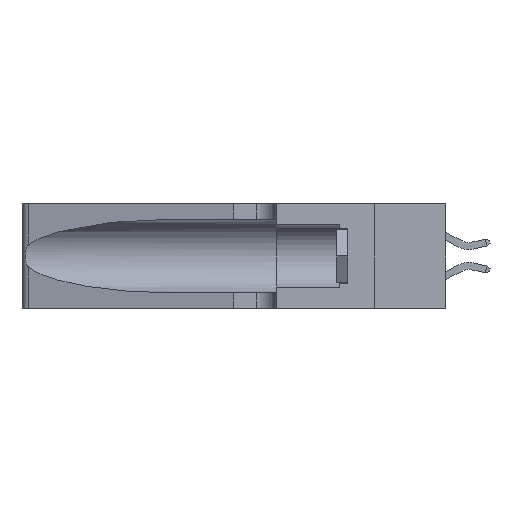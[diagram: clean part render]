
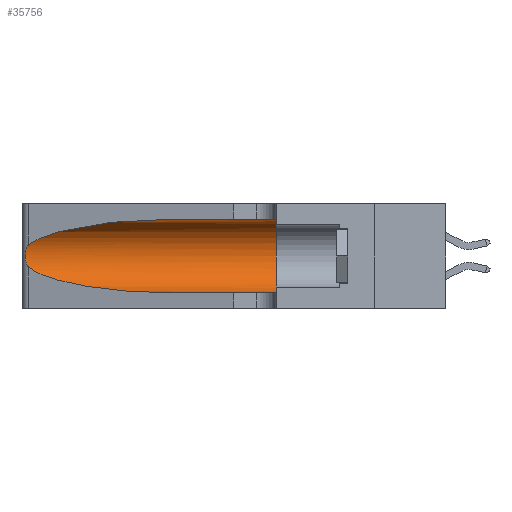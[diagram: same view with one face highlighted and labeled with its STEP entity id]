
A CAD part, left-side view. The second image highlights one B-rep face of the part: STEP entity #35756.
In plain terms, the highlighted cylindrical face has radius 3.308 mm (diameter 6.617 mm), a partial arc.
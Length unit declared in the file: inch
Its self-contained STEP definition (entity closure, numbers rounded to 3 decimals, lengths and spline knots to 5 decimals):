
#1296 = CARTESIAN_POINT ( 'NONE',  ( 0.1305, 0.35, 0.05475 ) ) ;
#1552 = AXIS2_PLACEMENT_3D ( 'NONE', #14078, #30241, #23945 ) ;
#2430 = CIRCLE ( 'NONE', #23096, 0.13025 ) ;
#2552 = LINE ( 'NONE', #2941, #21066 ) ;
#2925 = B_SPLINE_CURVE_WITH_KNOTS ( 'NONE', 3,
 ( #22454, #41890, #25480, #5813, #9516, #12143, #28913, #18743, #5947, #29052, #25911, #32332, #42167, #8942 ),
 .UNSPECIFIED., .F., .F.,
 ( 4, 2, 2, 2, 2, 2, 4 ),
 ( 0., 0.00027, 0.00053, 0.00107, 0.0016, 0.00187, 0.00214 ),
 .UNSPECIFIED. ) ;
#2941 = CARTESIAN_POINT ( 'NONE',  ( 0.1305, 1.61858, 0.31525 ) ) ;
#4139 = LINE ( 'NONE', #41108, #29340 ) ;
#5813 = CARTESIAN_POINT ( 'NONE',  ( 0.25787, 1.23484, 0.2124 ) ) ;
#5856 = ORIENTED_EDGE ( 'NONE', *, *, #32194, .T. ) ;
#5947 = CARTESIAN_POINT ( 'NONE',  ( 0.26017, 1.23833, 0.17102 ) ) ;
#8314 = DIRECTION ( 'NONE',  ( 0., 1., 0. ) ) ;
#8377 = CARTESIAN_POINT ( 'NONE',  ( 0.2373, 1.15595, 0.08982 ) ) ;
#8492 = EDGE_CURVE ( 'NONE', #18791, #25860, #2552, .T. ) ;
#8682 =( BOUNDED_CURVE ( )  B_SPLINE_CURVE ( 3, ( #11404, #37400, #37693, #36525 ),
 .UNSPECIFIED., .F., .T. ) 
 B_SPLINE_CURVE_WITH_KNOTS ( ( 4, 4 ),
 ( 1.5708, 2.84003 ),
 .UNSPECIFIED. ) 
 CURVE ( )  GEOMETRIC_REPRESENTATION_ITEM ( )  RATIONAL_B_SPLINE_CURVE ( ( 1., 0.87, 0.87, 1. ) ) 
 REPRESENTATION_ITEM ( '' )  );
#8942 = CARTESIAN_POINT ( 'NONE',  ( 0.25487, 1.22718, 0.14631 ) ) ;
#9205 = VERTEX_POINT ( 'NONE', #33877 ) ;
#9516 = CARTESIAN_POINT ( 'NONE',  ( 0.25854, 1.2359, 0.20912 ) ) ;
#10698 = EDGE_CURVE ( 'NONE', #9205, #23643, #28008, .T. ) ;
#11404 = CARTESIAN_POINT ( 'NONE',  ( 0.1305, 0.72297, 0.31525 ) ) ;
#11773 = CARTESIAN_POINT ( 'NONE',  ( 0.25487, 1.22718, 0.22369 ) ) ;
#12143 = CARTESIAN_POINT ( 'NONE',  ( 0.26018, 1.23835, 0.19895 ) ) ;
#12960 = ORIENTED_EDGE ( 'NONE', *, *, #31916, .T. ) ;
#13896 = ORIENTED_EDGE ( 'NONE', *, *, #37950, .T. ) ;
#14078 = CARTESIAN_POINT ( 'NONE',  ( 0.1305, 1.61858, 0.185 ) ) ;
#14563 = DIRECTION ( 'NONE',  ( 0., -1., 0. ) ) ;
#14567 = FACE_OUTER_BOUND ( 'NONE', #35007, .T. ) ;
#15566 = CYLINDRICAL_SURFACE ( 'NONE', #1552, 0.13025 ) ;
#18743 = CARTESIAN_POINT ( 'NONE',  ( 0.26075, 1.23896, 0.178 ) ) ;
#18791 = VERTEX_POINT ( 'NONE', #18945 ) ;
#18945 = CARTESIAN_POINT ( 'NONE',  ( 0.1305, 0.72297, 0.31525 ) ) ;
#21066 = VECTOR ( 'NONE', #14563, 39.37008 ) ;
#21091 = VERTEX_POINT ( 'NONE', #1296 ) ;
#21571 = DIRECTION ( 'NONE',  ( 0., 0., 1. ) ) ;
#21634 = CARTESIAN_POINT ( 'NONE',  ( 0.1305, 0.72297, 0.05475 ) ) ;
#22168 = CARTESIAN_POINT ( 'NONE',  ( 0.1305, 0.72297, 0.05475 ) ) ;
#22454 = CARTESIAN_POINT ( 'NONE',  ( 0.25487, 1.22718, 0.22369 ) ) ;
#23096 = AXIS2_PLACEMENT_3D ( 'NONE', #30112, #8314, #21571 ) ;
#23643 = VERTEX_POINT ( 'NONE', #21634 ) ;
#23945 = DIRECTION ( 'NONE',  ( 0., 0., -1. ) ) ;
#24528 = VERTEX_POINT ( 'NONE', #11773 ) ;
#24818 = ORIENTED_EDGE ( 'NONE', *, *, #29209, .F. ) ;
#25480 = CARTESIAN_POINT ( 'NONE',  ( 0.25639, 1.23184, 0.21858 ) ) ;
#25788 = ORIENTED_EDGE ( 'NONE', *, *, #8492, .F. ) ;
#25860 = VERTEX_POINT ( 'NONE', #30419 ) ;
#25911 = CARTESIAN_POINT ( 'NONE',  ( 0.25789, 1.23486, 0.15765 ) ) ;
#27796 = ORIENTED_EDGE ( 'NONE', *, *, #10698, .T. ) ;
#28008 =( BOUNDED_CURVE ( )  B_SPLINE_CURVE ( 3, ( #36034, #8377, #41450, #22168 ),
 .UNSPECIFIED., .F., .T. ) 
 B_SPLINE_CURVE_WITH_KNOTS ( ( 4, 4 ),
 ( 3.44316, 4.71239 ),
 .UNSPECIFIED. ) 
 CURVE ( )  GEOMETRIC_REPRESENTATION_ITEM ( )  RATIONAL_B_SPLINE_CURVE ( ( 1., 0.87, 0.87, 1. ) ) 
 REPRESENTATION_ITEM ( '' )  );
#28913 = CARTESIAN_POINT ( 'NONE',  ( 0.26075, 1.23896, 0.19203 ) ) ;
#29052 = CARTESIAN_POINT ( 'NONE',  ( 0.25856, 1.23593, 0.16098 ) ) ;
#29209 = EDGE_CURVE ( 'NONE', #25860, #21091, #2430, .T. ) ;
#29340 = VECTOR ( 'NONE', #35046, 39.37008 ) ;
#30112 = CARTESIAN_POINT ( 'NONE',  ( 0.1305, 0.35, 0.185 ) ) ;
#30241 = DIRECTION ( 'NONE',  ( 0., -1., 0. ) ) ;
#30419 = CARTESIAN_POINT ( 'NONE',  ( 0.1305, 0.35, 0.31525 ) ) ;
#31916 = EDGE_CURVE ( 'NONE', #24528, #9205, #2925, .T. ) ;
#32194 = EDGE_CURVE ( 'NONE', #18791, #24528, #8682, .T. ) ;
#32332 = CARTESIAN_POINT ( 'NONE',  ( 0.25639, 1.23186, 0.15144 ) ) ;
#33877 = CARTESIAN_POINT ( 'NONE',  ( 0.25487, 1.22718, 0.14631 ) ) ;
#35007 = EDGE_LOOP ( 'NONE', ( #5856, #12960, #27796, #13896, #24818, #25788 ) ) ;
#35046 = DIRECTION ( 'NONE',  ( 0., -1., 0. ) ) ;
#35756 = ADVANCED_FACE ( 'NONE', ( #14567 ), #15566, .F. ) ;
#36034 = CARTESIAN_POINT ( 'NONE',  ( 0.25487, 1.22718, 0.14631 ) ) ;
#36525 = CARTESIAN_POINT ( 'NONE',  ( 0.25487, 1.22718, 0.22369 ) ) ;
#37400 = CARTESIAN_POINT ( 'NONE',  ( 0.18966, 0.96281, 0.31525 ) ) ;
#37693 = CARTESIAN_POINT ( 'NONE',  ( 0.2373, 1.15595, 0.28018 ) ) ;
#37950 = EDGE_CURVE ( 'NONE', #23643, #21091, #4139, .T. ) ;
#41108 = CARTESIAN_POINT ( 'NONE',  ( 0.1305, 1.61858, 0.05475 ) ) ;
#41450 = CARTESIAN_POINT ( 'NONE',  ( 0.18966, 0.96281, 0.05475 ) ) ;
#41890 = CARTESIAN_POINT ( 'NONE',  ( 0.25555, 1.22994, 0.2215 ) ) ;
#42167 = CARTESIAN_POINT ( 'NONE',  ( 0.25555, 1.22993, 0.14849 ) ) ;
